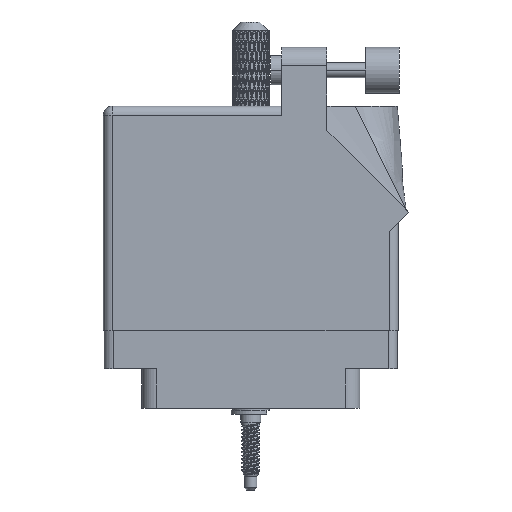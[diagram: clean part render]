
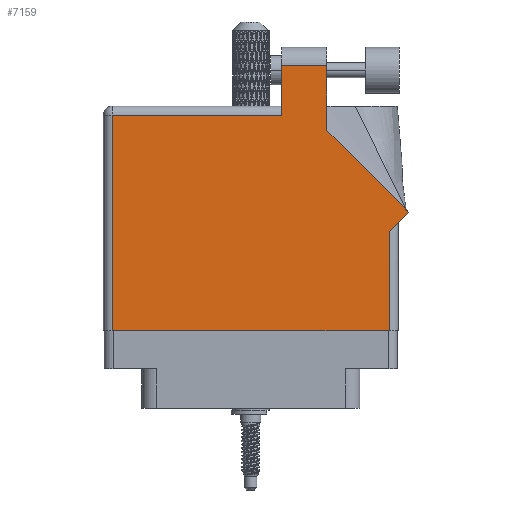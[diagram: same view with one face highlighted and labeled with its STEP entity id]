
A CAD part, front view. The second image highlights one B-rep face of the part: STEP entity #7159.
In plain terms, the highlighted face is planar.
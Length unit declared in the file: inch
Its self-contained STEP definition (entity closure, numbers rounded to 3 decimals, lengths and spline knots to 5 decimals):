
#785 = CARTESIAN_POINT ( 'NONE',  ( 1.948, 0.675, 0. ) ) ;
#868 = EDGE_LOOP ( 'NONE', ( #89867, #16937, #31606, #2064, #71191, #58415, #11265, #51577, #49500 ) ) ;
#1792 = DIRECTION ( 'NONE',  ( 1., 0., 0. ) ) ;
#2064 = ORIENTED_EDGE ( 'NONE', *, *, #87681, .T. ) ;
#3865 = LINE ( 'NONE', #52099, #15642 ) ;
#4814 = LINE ( 'NONE', #84839, #30725 ) ;
#7159 = ADVANCED_FACE ( 'NONE', ( #101950 ), #29358, .F. ) ;
#7919 = VECTOR ( 'NONE', #35814, 39.37008 ) ;
#10246 = DIRECTION ( 'NONE',  ( 0., -1., 0. ) ) ;
#11265 = ORIENTED_EDGE ( 'NONE', *, *, #67082, .T. ) ;
#12475 = LINE ( 'NONE', #44803, #55386 ) ;
#12967 = VERTEX_POINT ( 'NONE', #83275 ) ;
#13550 = CARTESIAN_POINT ( 'NONE',  ( 1.948, 0., 0. ) ) ;
#14437 = LINE ( 'NONE', #46762, #92381 ) ;
#15642 = VECTOR ( 'NONE', #10246, 39.37008 ) ;
#16351 = EDGE_CURVE ( 'NONE', #103097, #46220, #80201, .T. ) ;
#16690 = CARTESIAN_POINT ( 'NONE',  ( 1.217, 1.468, 0. ) ) ;
#16937 = ORIENTED_EDGE ( 'NONE', *, *, #51466, .T. ) ;
#17370 = EDGE_CURVE ( 'NONE', #52042, #12967, #36122, .T. ) ;
#18929 = VERTEX_POINT ( 'NONE', #16690 ) ;
#20878 = DIRECTION ( 'NONE',  ( -1., 0., 0. ) ) ;
#21395 = DIRECTION ( 'NONE',  ( 0., 0., -1. ) ) ;
#23560 = EDGE_CURVE ( 'NONE', #43543, #44605, #14437, .T. ) ;
#29358 = PLANE ( 'NONE',  #58010 ) ;
#30725 = VECTOR ( 'NONE', #76358, 39.37008 ) ;
#31606 = ORIENTED_EDGE ( 'NONE', *, *, #95205, .T. ) ;
#35814 = DIRECTION ( 'NONE',  ( -1., 0., 0. ) ) ;
#36122 = LINE ( 'NONE', #100738, #97690 ) ;
#36659 = CARTESIAN_POINT ( 'NONE',  ( 2.08071, 0.80771, 0. ) ) ;
#38359 = VECTOR ( 'NONE', #39892, 39.37008 ) ;
#39892 = DIRECTION ( 'NONE',  ( 0.707, 0.707, 0. ) ) ;
#40408 = CARTESIAN_POINT ( 'NONE',  ( 1.524, 1.36442, 0. ) ) ;
#43543 = VERTEX_POINT ( 'NONE', #49743 ) ;
#44605 = VERTEX_POINT ( 'NONE', #99690 ) ;
#44803 = CARTESIAN_POINT ( 'NONE',  ( 1.948, 0.737, 0. ) ) ;
#46220 = VERTEX_POINT ( 'NONE', #36659 ) ;
#46680 = EDGE_CURVE ( 'NONE', #46220, #52042, #83012, .T. ) ;
#46762 = CARTESIAN_POINT ( 'NONE',  ( 0.062, 0., 0. ) ) ;
#49500 = ORIENTED_EDGE ( 'NONE', *, *, #46680, .T. ) ;
#49743 = CARTESIAN_POINT ( 'NONE',  ( 0.062, 1.468, 0. ) ) ;
#51466 = EDGE_CURVE ( 'NONE', #12967, #53264, #68641, .T. ) ;
#51577 = ORIENTED_EDGE ( 'NONE', *, *, #16351, .T. ) ;
#52042 = VERTEX_POINT ( 'NONE', #40408 ) ;
#52099 = CARTESIAN_POINT ( 'NONE',  ( 1.217, 1.53, 0. ) ) ;
#52233 = DIRECTION ( 'NONE',  ( 0., 1., 0. ) ) ;
#53264 = VERTEX_POINT ( 'NONE', #75547 ) ;
#54091 = DIRECTION ( 'NONE',  ( 0., 1., 0. ) ) ;
#55386 = VECTOR ( 'NONE', #52233, 39.37008 ) ;
#58010 = AXIS2_PLACEMENT_3D ( 'NONE', #61680, #21395, #20878 ) ;
#58415 = ORIENTED_EDGE ( 'NONE', *, *, #103742, .T. ) ;
#61680 = CARTESIAN_POINT ( 'NONE',  ( 0., 1.53, 0. ) ) ;
#66600 = CARTESIAN_POINT ( 'NONE',  ( 2.08071, 0.80771, 0. ) ) ;
#67082 = EDGE_CURVE ( 'NONE', #89807, #103097, #12475, .T. ) ;
#68641 = LINE ( 'NONE', #101495, #7919 ) ;
#71191 = ORIENTED_EDGE ( 'NONE', *, *, #23560, .T. ) ;
#73266 = CARTESIAN_POINT ( 'NONE',  ( 2.01, 0.737, 0. ) ) ;
#75547 = CARTESIAN_POINT ( 'NONE',  ( 1.217, 1.805, 0. ) ) ;
#76358 = DIRECTION ( 'NONE',  ( -1., 0., 0. ) ) ;
#77912 = LINE ( 'NONE', #82357, #92319 ) ;
#80201 = LINE ( 'NONE', #73266, #38359 ) ;
#82357 = CARTESIAN_POINT ( 'NONE',  ( 0., 0., 0. ) ) ;
#83012 = LINE ( 'NONE', #66600, #95812 ) ;
#83275 = CARTESIAN_POINT ( 'NONE',  ( 1.524, 1.805, 0. ) ) ;
#84839 = CARTESIAN_POINT ( 'NONE',  ( 0., 1.468, 0. ) ) ;
#87681 = EDGE_CURVE ( 'NONE', #18929, #43543, #4814, .T. ) ;
#89807 = VERTEX_POINT ( 'NONE', #13550 ) ;
#89867 = ORIENTED_EDGE ( 'NONE', *, *, #17370, .T. ) ;
#92319 = VECTOR ( 'NONE', #1792, 39.37008 ) ;
#92381 = VECTOR ( 'NONE', #96567, 39.37008 ) ;
#95205 = EDGE_CURVE ( 'NONE', #53264, #18929, #3865, .T. ) ;
#95812 = VECTOR ( 'NONE', #98380, 39.37008 ) ;
#96567 = DIRECTION ( 'NONE',  ( 0., -1., 0. ) ) ;
#97690 = VECTOR ( 'NONE', #54091, 39.37008 ) ;
#98380 = DIRECTION ( 'NONE',  ( -0.707, 0.707, 0. ) ) ;
#99690 = CARTESIAN_POINT ( 'NONE',  ( 0.062, 0., 0. ) ) ;
#100738 = CARTESIAN_POINT ( 'NONE',  ( 1.524, 1.36442, 0. ) ) ;
#101495 = CARTESIAN_POINT ( 'NONE',  ( 1.217, 1.805, 0. ) ) ;
#101950 = FACE_OUTER_BOUND ( 'NONE', #868, .T. ) ;
#103097 = VERTEX_POINT ( 'NONE', #785 ) ;
#103742 = EDGE_CURVE ( 'NONE', #44605, #89807, #77912, .T. ) ;
